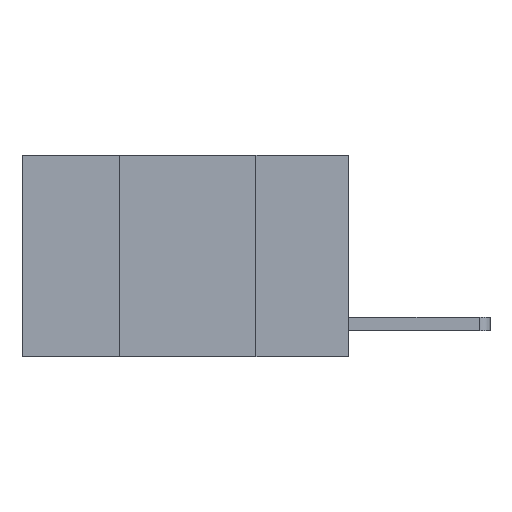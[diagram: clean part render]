
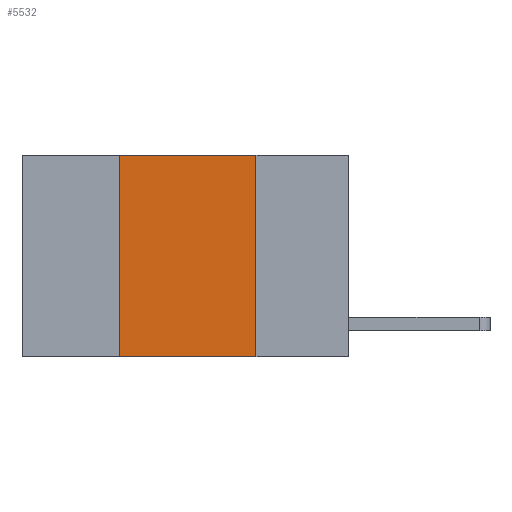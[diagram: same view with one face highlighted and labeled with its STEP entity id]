
A CAD part, left-side view. The second image highlights one B-rep face of the part: STEP entity #5532.
In plain terms, the highlighted planar face has unit normal (-1, 0, 0).
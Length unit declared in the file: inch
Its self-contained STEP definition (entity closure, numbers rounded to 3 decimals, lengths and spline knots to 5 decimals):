
#77 = VECTOR ( 'NONE', #7899, 39.37008 ) ;
#500 = VERTEX_POINT ( 'NONE', #654 ) ;
#654 = CARTESIAN_POINT ( 'NONE',  ( 0., 0.17, 0. ) ) ;
#806 = VECTOR ( 'NONE', #3762, 39.37008 ) ;
#827 = EDGE_CURVE ( 'NONE', #4408, #9045, #9477, .T. ) ;
#1176 = PLANE ( 'NONE',  #2658 ) ;
#2238 = LINE ( 'NONE', #6656, #6053 ) ;
#2283 = CARTESIAN_POINT ( 'NONE',  ( 0., 0.42, -0.37 ) ) ;
#2394 = EDGE_LOOP ( 'NONE', ( #6174, #5125, #6575, #7660 ) ) ;
#2520 = CARTESIAN_POINT ( 'NONE',  ( 0., 0.17, -0.37 ) ) ;
#2658 = AXIS2_PLACEMENT_3D ( 'NONE', #4286, #9326, #5029 ) ;
#3033 = CARTESIAN_POINT ( 'NONE',  ( 0., 0.42, 0. ) ) ;
#3060 = FACE_OUTER_BOUND ( 'NONE', #2394, .T. ) ;
#3762 = DIRECTION ( 'NONE',  ( 0., -1., 0. ) ) ;
#3930 = EDGE_CURVE ( 'NONE', #4408, #7679, #7470, .T. ) ;
#4286 = CARTESIAN_POINT ( 'NONE',  ( 0., 0.6, 0. ) ) ;
#4408 = VERTEX_POINT ( 'NONE', #2283 ) ;
#5029 = DIRECTION ( 'NONE',  ( 0., 0., -1. ) ) ;
#5125 = ORIENTED_EDGE ( 'NONE', *, *, #8291, .F. ) ;
#5532 = ADVANCED_FACE ( 'NONE', ( #3060 ), #1176, .F. ) ;
#5576 = DIRECTION ( 'NONE',  ( 0., 0., 1. ) ) ;
#5673 = EDGE_CURVE ( 'NONE', #500, #9045, #2238, .T. ) ;
#5903 = DIRECTION ( 'NONE',  ( 0., 0., -1. ) ) ;
#6053 = VECTOR ( 'NONE', #5903, 39.37008 ) ;
#6174 = ORIENTED_EDGE ( 'NONE', *, *, #5673, .F. ) ;
#6575 = ORIENTED_EDGE ( 'NONE', *, *, #3930, .F. ) ;
#6656 = CARTESIAN_POINT ( 'NONE',  ( 0., 0.17, 0. ) ) ;
#6864 = LINE ( 'NONE', #9579, #806 ) ;
#7028 = CARTESIAN_POINT ( 'NONE',  ( 0., 0.6, -0.37 ) ) ;
#7470 = LINE ( 'NONE', #9151, #9084 ) ;
#7660 = ORIENTED_EDGE ( 'NONE', *, *, #827, .T. ) ;
#7679 = VERTEX_POINT ( 'NONE', #3033 ) ;
#7899 = DIRECTION ( 'NONE',  ( 0., -1., 0. ) ) ;
#8291 = EDGE_CURVE ( 'NONE', #7679, #500, #6864, .T. ) ;
#9045 = VERTEX_POINT ( 'NONE', #2520 ) ;
#9084 = VECTOR ( 'NONE', #5576, 39.37008 ) ;
#9151 = CARTESIAN_POINT ( 'NONE',  ( 0., 0.42, 0. ) ) ;
#9326 = DIRECTION ( 'NONE',  ( 1., 0., 0. ) ) ;
#9477 = LINE ( 'NONE', #7028, #77 ) ;
#9579 = CARTESIAN_POINT ( 'NONE',  ( 0., 0.6, 0. ) ) ;
